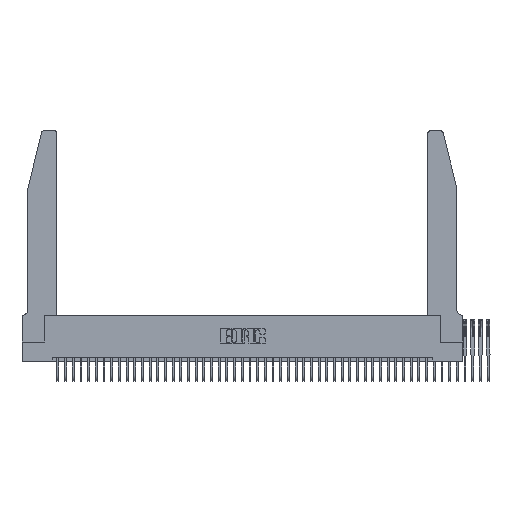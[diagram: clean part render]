
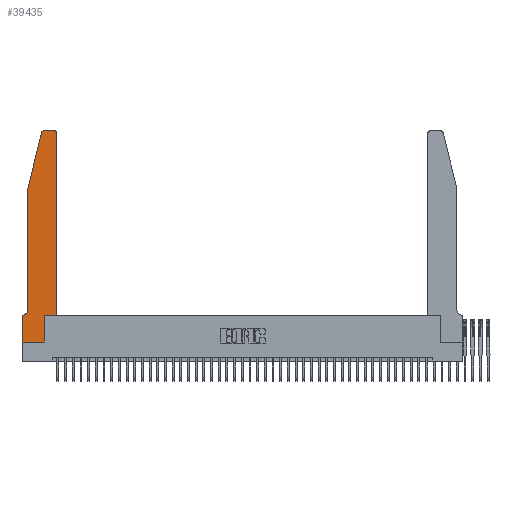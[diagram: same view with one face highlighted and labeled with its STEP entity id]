
A CAD part, top view. The second image highlights one B-rep face of the part: STEP entity #39435.
In plain terms, the highlighted planar face has unit normal (0, 0, 1).
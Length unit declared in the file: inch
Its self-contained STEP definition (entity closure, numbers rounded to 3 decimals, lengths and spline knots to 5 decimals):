
#795 = CARTESIAN_POINT ( 'NONE',  ( 0.25487, 2.72718, 0.37 ) ) ;
#963 = DIRECTION ( 'NONE',  ( 0., 0., 1. ) ) ;
#1382 = ORIENTED_EDGE ( 'NONE', *, *, #1792, .T. ) ;
#1792 = EDGE_CURVE ( 'NONE', #31449, #40930, #37029, .T. ) ;
#1831 = EDGE_CURVE ( 'NONE', #35921, #31449, #27745, .T. ) ;
#4027 = EDGE_CURVE ( 'NONE', #40930, #29914, #23906, .T. ) ;
#5903 = DIRECTION ( 'NONE',  ( 1., 0., 0. ) ) ;
#6263 = VERTEX_POINT ( 'NONE', #32356 ) ;
#6646 = CARTESIAN_POINT ( 'NONE',  ( 0.0755, 0.35, 0.37 ) ) ;
#7644 = VERTEX_POINT ( 'NONE', #20789 ) ;
#8557 = DIRECTION ( 'NONE',  ( 0., 1., 0. ) ) ;
#8708 = AXIS2_PLACEMENT_3D ( 'NONE', #15131, #37038, #18287 ) ;
#9622 = EDGE_CURVE ( 'NONE', #19281, #12524, #35653, .T. ) ;
#9648 = VECTOR ( 'NONE', #28048, 39.37008 ) ;
#10241 = ORIENTED_EDGE ( 'NONE', *, *, #24059, .T. ) ;
#10546 = CARTESIAN_POINT ( 'NONE',  ( 0.0755, 2., 0.37 ) ) ;
#10656 = LINE ( 'NONE', #18711, #9648 ) ;
#11213 = EDGE_CURVE ( 'NONE', #29914, #35776, #29684, .T. ) ;
#11245 = CARTESIAN_POINT ( 'NONE',  ( 0.2865, 0.35, 0.37 ) ) ;
#11953 = VECTOR ( 'NONE', #13174, 39.37008 ) ;
#11967 = VECTOR ( 'NONE', #8557, 39.37008 ) ;
#12524 = VERTEX_POINT ( 'NONE', #33633 ) ;
#12576 = EDGE_CURVE ( 'NONE', #37130, #19281, #28610, .T. ) ;
#12702 = EDGE_CURVE ( 'NONE', #35776, #35025, #24692, .T. ) ;
#12991 = LINE ( 'NONE', #30660, #11967 ) ;
#13174 = DIRECTION ( 'NONE',  ( -1., 0., 0. ) ) ;
#13571 = ORIENTED_EDGE ( 'NONE', *, *, #40480, .T. ) ;
#13638 = LINE ( 'NONE', #33341, #21039 ) ;
#13753 = EDGE_LOOP ( 'NONE', ( #13571, #14182, #40826, #39442, #14757, #1382, #16212, #27352, #22647, #10241, #28039, #25422 ) ) ;
#13791 = DIRECTION ( 'NONE',  ( -0.239, -0.971, 0. ) ) ;
#14182 = ORIENTED_EDGE ( 'NONE', *, *, #12576, .T. ) ;
#14509 = CARTESIAN_POINT ( 'NONE',  ( 0., 0., 0.37 ) ) ;
#14724 = EDGE_CURVE ( 'NONE', #6263, #36712, #26967, .T. ) ;
#14757 = ORIENTED_EDGE ( 'NONE', *, *, #1831, .T. ) ;
#15118 = CARTESIAN_POINT ( 'NONE',  ( 0., 0.35, 0.37 ) ) ;
#15131 = CARTESIAN_POINT ( 'NONE',  ( 0.284, 2.72, 0.37 ) ) ;
#16212 = ORIENTED_EDGE ( 'NONE', *, *, #4027, .T. ) ;
#16476 = CARTESIAN_POINT ( 'NONE',  ( 0., 0., 0.37 ) ) ;
#16489 = DIRECTION ( 'NONE',  ( 0., 0., -1. ) ) ;
#16715 = DIRECTION ( 'NONE',  ( 0., 0., 1. ) ) ;
#16800 = AXIS2_PLACEMENT_3D ( 'NONE', #35478, #16715, #38611 ) ;
#16991 = PLANE ( 'NONE',  #37226 ) ;
#18022 = VECTOR ( 'NONE', #13791, 39.37008 ) ;
#18287 = DIRECTION ( 'NONE',  ( 1., 0., 0. ) ) ;
#18711 = CARTESIAN_POINT ( 'NONE',  ( 0.2605, 2.75, 0.37 ) ) ;
#19281 = VERTEX_POINT ( 'NONE', #795 ) ;
#20151 = CARTESIAN_POINT ( 'NONE',  ( 0., 0.35, 0.37 ) ) ;
#20789 = CARTESIAN_POINT ( 'NONE',  ( 0.4505, 0.35, 0.37 ) ) ;
#21039 = VECTOR ( 'NONE', #36485, 39.37008 ) ;
#22647 = ORIENTED_EDGE ( 'NONE', *, *, #12702, .T. ) ;
#23294 = DIRECTION ( 'NONE',  ( 1., 0., 0. ) ) ;
#23694 = VECTOR ( 'NONE', #28169, 39.37008 ) ;
#23906 = LINE ( 'NONE', #14509, #39552 ) ;
#24059 = EDGE_CURVE ( 'NONE', #35025, #7644, #25418, .T. ) ;
#24301 = CARTESIAN_POINT ( 'NONE',  ( 0.4205, 2.75, 0.37 ) ) ;
#24692 = LINE ( 'NONE', #25027, #23694 ) ;
#24985 = CARTESIAN_POINT ( 'NONE',  ( 0.4505, 0.35, 0.37 ) ) ;
#25027 = CARTESIAN_POINT ( 'NONE',  ( 0.2865, 0.35, 0.37 ) ) ;
#25418 = LINE ( 'NONE', #24985, #33712 ) ;
#25422 = ORIENTED_EDGE ( 'NONE', *, *, #14724, .T. ) ;
#25964 = AXIS2_PLACEMENT_3D ( 'NONE', #35258, #16489, #38388 ) ;
#26967 = CIRCLE ( 'NONE', #16800, 0.03 ) ;
#27352 = ORIENTED_EDGE ( 'NONE', *, *, #11213, .T. ) ;
#27745 = CIRCLE ( 'NONE', #25964, 0.07 ) ;
#28039 = ORIENTED_EDGE ( 'NONE', *, *, #39260, .T. ) ;
#28048 = DIRECTION ( 'NONE',  ( -1., 0., 0. ) ) ;
#28169 = DIRECTION ( 'NONE',  ( 0., 1., 0. ) ) ;
#28610 = CIRCLE ( 'NONE', #8708, 0.03 ) ;
#29196 = CARTESIAN_POINT ( 'NONE',  ( 0.0055, 0.35, 0.37 ) ) ;
#29684 = LINE ( 'NONE', #16476, #30668 ) ;
#29914 = VERTEX_POINT ( 'NONE', #30995 ) ;
#30660 = CARTESIAN_POINT ( 'NONE',  ( 0.4505, 0.35, 0.37 ) ) ;
#30668 = VECTOR ( 'NONE', #38378, 39.37008 ) ;
#30995 = CARTESIAN_POINT ( 'NONE',  ( 0., 0., 0.37 ) ) ;
#30999 = EDGE_CURVE ( 'NONE', #12524, #35921, #13638, .T. ) ;
#31449 = VERTEX_POINT ( 'NONE', #29196 ) ;
#32356 = CARTESIAN_POINT ( 'NONE',  ( 0.4505, 2.72, 0.37 ) ) ;
#33284 = DIRECTION ( 'NONE',  ( 0., -1., 0. ) ) ;
#33341 = CARTESIAN_POINT ( 'NONE',  ( 0.0755, 2., 0.37 ) ) ;
#33633 = CARTESIAN_POINT ( 'NONE',  ( 0.0755, 2., 0.37 ) ) ;
#33712 = VECTOR ( 'NONE', #5903, 39.37008 ) ;
#34573 = CARTESIAN_POINT ( 'NONE',  ( 0.0755, 0.42, 0.37 ) ) ;
#35025 = VERTEX_POINT ( 'NONE', #11245 ) ;
#35258 = CARTESIAN_POINT ( 'NONE',  ( 0.0055, 0.42, 0.37 ) ) ;
#35478 = CARTESIAN_POINT ( 'NONE',  ( 0.4205, 2.72, 0.37 ) ) ;
#35601 = CARTESIAN_POINT ( 'NONE',  ( 0.284, 2.75, 0.37 ) ) ;
#35653 = LINE ( 'NONE', #10546, #18022 ) ;
#35776 = VERTEX_POINT ( 'NONE', #37045 ) ;
#35921 = VERTEX_POINT ( 'NONE', #34573 ) ;
#36485 = DIRECTION ( 'NONE',  ( 0., -1., 0. ) ) ;
#36712 = VERTEX_POINT ( 'NONE', #24301 ) ;
#37029 = LINE ( 'NONE', #6646, #11953 ) ;
#37038 = DIRECTION ( 'NONE',  ( 0., 0., 1. ) ) ;
#37045 = CARTESIAN_POINT ( 'NONE',  ( 0.2865, 0., 0.37 ) ) ;
#37130 = VERTEX_POINT ( 'NONE', #35601 ) ;
#37226 = AXIS2_PLACEMENT_3D ( 'NONE', #20151, #963, #23294 ) ;
#38378 = DIRECTION ( 'NONE',  ( 1., 0., 0. ) ) ;
#38388 = DIRECTION ( 'NONE',  ( -1., 0., 0. ) ) ;
#38481 = FACE_OUTER_BOUND ( 'NONE', #13753, .T. ) ;
#38611 = DIRECTION ( 'NONE',  ( 1., 0., 0. ) ) ;
#39260 = EDGE_CURVE ( 'NONE', #7644, #6263, #12991, .T. ) ;
#39435 = ADVANCED_FACE ( 'NONE', ( #38481 ), #16991, .T. ) ;
#39442 = ORIENTED_EDGE ( 'NONE', *, *, #30999, .T. ) ;
#39552 = VECTOR ( 'NONE', #33284, 39.37008 ) ;
#40480 = EDGE_CURVE ( 'NONE', #36712, #37130, #10656, .T. ) ;
#40826 = ORIENTED_EDGE ( 'NONE', *, *, #9622, .T. ) ;
#40930 = VERTEX_POINT ( 'NONE', #15118 ) ;
